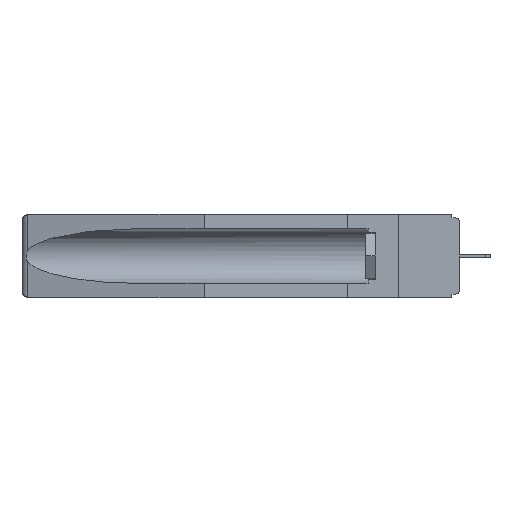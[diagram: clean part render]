
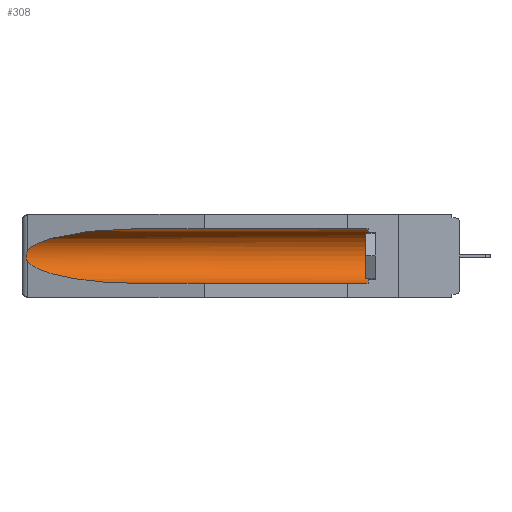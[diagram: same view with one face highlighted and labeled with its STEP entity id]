
A CAD part, left-side view. The second image highlights one B-rep face of the part: STEP entity #308.
In plain terms, the highlighted cylindrical face has radius 2.857 mm (diameter 5.715 mm), a partial arc.
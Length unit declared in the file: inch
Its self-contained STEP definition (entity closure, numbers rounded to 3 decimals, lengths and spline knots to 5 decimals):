
#35 = B_SPLINE_CURVE_WITH_KNOTS ( 'NONE', 3,
 ( #10363, #8998, #11764, #3675, #13115, #5022, #14441, #6374, #15782, #7714 ),
 .UNSPECIFIED., .F., .F.,
 ( 4, 2, 2, 2, 4 ),
 ( 0., 0.00029, 0.00058, 0.00087, 0.00117 ),
 .UNSPECIFIED. ) ;
#308 = ADVANCED_FACE ( 'NONE', ( #6206 ), #5786, .F. ) ;
#418 = ORIENTED_EDGE ( 'NONE', *, *, #5376, .T. ) ;
#482 = CARTESIAN_POINT ( 'NONE',  ( 0.155, 0.126, -0.284 ) ) ;
#918 = EDGE_CURVE ( 'NONE', #16884, #5468, #8248, .T. ) ;
#1491 = AXIS2_PLACEMENT_3D ( 'NONE', #14550, #6474, #15887 ) ;
#1547 = AXIS2_PLACEMENT_3D ( 'NONE', #2566, #2277, #8365 ) ;
#2277 = DIRECTION ( 'NONE',  ( 0., 1., 0. ) ) ;
#2528 =( BOUNDED_CURVE ( )  B_SPLINE_CURVE ( 3, ( #3553, #7594, #13040, #4959 ),
 .UNSPECIFIED., .F., .F. ) 
 B_SPLINE_CURVE_WITH_KNOTS ( ( 4, 4 ),
 ( 4.71239, 6.08839 ),
 .UNSPECIFIED. ) 
 CURVE ( )  GEOMETRIC_REPRESENTATION_ITEM ( )  RATIONAL_B_SPLINE_CURVE ( ( 1., 0.848, 0.848, 1. ) ) 
 REPRESENTATION_ITEM ( '' )  );
#2566 = CARTESIAN_POINT ( 'NONE',  ( 0.155, -0.30754, -0.1715 ) ) ;
#2602 = VERTEX_POINT ( 'NONE', #11420 ) ;
#3192 = CARTESIAN_POINT ( 'NONE',  ( 0.21114, 1.30732, -0.284 ) ) ;
#3553 = CARTESIAN_POINT ( 'NONE',  ( 0.155, 1.07973, -0.059 ) ) ;
#3661 = CARTESIAN_POINT ( 'NONE',  ( 0.155, 1.07973, -0.059 ) ) ;
#3675 = CARTESIAN_POINT ( 'NONE',  ( 0.2673, 1.5327, -0.16383 ) ) ;
#3689 = ORIENTED_EDGE ( 'NONE', *, *, #15114, .T. ) ;
#3740 = ORIENTED_EDGE ( 'NONE', *, *, #10896, .F. ) ;
#4436 = EDGE_CURVE ( 'NONE', #2602, #9497, #15044, .T. ) ;
#4898 = CARTESIAN_POINT ( 'NONE',  ( 0.25451, 1.48313, -0.24835 ) ) ;
#4959 = CARTESIAN_POINT ( 'NONE',  ( 0.26537, 1.52718, -0.14972 ) ) ;
#5022 = CARTESIAN_POINT ( 'NONE',  ( 0.2675, 1.53308, -0.17534 ) ) ;
#5091 = ORIENTED_EDGE ( 'NONE', *, *, #15191, .T. ) ;
#5251 = VERTEX_POINT ( 'NONE', #16597 ) ;
#5376 = EDGE_CURVE ( 'NONE', #5251, #16884, #35, .T. ) ;
#5468 = VERTEX_POINT ( 'NONE', #15959 ) ;
#5786 = CYLINDRICAL_SURFACE ( 'NONE', #1547, 0.1125 ) ;
#6206 = FACE_OUTER_BOUND ( 'NONE', #17355, .T. ) ;
#6374 = CARTESIAN_POINT ( 'NONE',  ( 0.26655, 1.53094, -0.18657 ) ) ;
#6474 = DIRECTION ( 'NONE',  ( 0., -1., 0. ) ) ;
#6485 = LINE ( 'NONE', #14271, #13250 ) ;
#7594 = CARTESIAN_POINT ( 'NONE',  ( 0.21114, 1.30732, -0.059 ) ) ;
#7714 = CARTESIAN_POINT ( 'NONE',  ( 0.26537, 1.52718, -0.19328 ) ) ;
#8248 =( BOUNDED_CURVE ( )  B_SPLINE_CURVE ( 3, ( #9800, #4898, #3192, #9164 ),
 .UNSPECIFIED., .F., .F. ) 
 B_SPLINE_CURVE_WITH_KNOTS ( ( 4, 4 ),
 ( 0.1948, 1.5708 ),
 .UNSPECIFIED. ) 
 CURVE ( )  GEOMETRIC_REPRESENTATION_ITEM ( )  RATIONAL_B_SPLINE_CURVE ( ( 1., 0.848, 0.848, 1. ) ) 
 REPRESENTATION_ITEM ( '' )  );
#8365 = DIRECTION ( 'NONE',  ( 0., 0., 1. ) ) ;
#8998 = CARTESIAN_POINT ( 'NONE',  ( 0.26597, 1.52961, -0.15275 ) ) ;
#9164 = CARTESIAN_POINT ( 'NONE',  ( 0.155, 1.07973, -0.284 ) ) ;
#9497 = VERTEX_POINT ( 'NONE', #3661 ) ;
#9800 = CARTESIAN_POINT ( 'NONE',  ( 0.26537, 1.52718, -0.19328 ) ) ;
#10363 = CARTESIAN_POINT ( 'NONE',  ( 0.26537, 1.52718, -0.14972 ) ) ;
#10792 = VERTEX_POINT ( 'NONE', #482 ) ;
#10896 = EDGE_CURVE ( 'NONE', #10792, #5468, #6485, .T. ) ;
#11054 = VECTOR ( 'NONE', #14106, 39.37008 ) ;
#11420 = CARTESIAN_POINT ( 'NONE',  ( 0.155, 0.126, -0.059 ) ) ;
#11439 = CIRCLE ( 'NONE', #1491, 0.1125 ) ;
#11764 = CARTESIAN_POINT ( 'NONE',  ( 0.26654, 1.53092, -0.15636 ) ) ;
#12186 = ORIENTED_EDGE ( 'NONE', *, *, #918, .T. ) ;
#13040 = CARTESIAN_POINT ( 'NONE',  ( 0.25451, 1.48313, -0.09465 ) ) ;
#13115 = CARTESIAN_POINT ( 'NONE',  ( 0.2675, 1.53308, -0.16763 ) ) ;
#13250 = VECTOR ( 'NONE', #15606, 39.37008 ) ;
#14063 = CARTESIAN_POINT ( 'NONE',  ( 0.155, -0.30754, -0.059 ) ) ;
#14106 = DIRECTION ( 'NONE',  ( 0., 1., 0. ) ) ;
#14271 = CARTESIAN_POINT ( 'NONE',  ( 0.155, -0.30754, -0.284 ) ) ;
#14441 = CARTESIAN_POINT ( 'NONE',  ( 0.2673, 1.53269, -0.17917 ) ) ;
#14550 = CARTESIAN_POINT ( 'NONE',  ( 0.155, 0.126, -0.1715 ) ) ;
#14930 = CARTESIAN_POINT ( 'NONE',  ( 0.26537, 1.52718, -0.19328 ) ) ;
#15044 = LINE ( 'NONE', #14063, #11054 ) ;
#15114 = EDGE_CURVE ( 'NONE', #9497, #5251, #2528, .T. ) ;
#15191 = EDGE_CURVE ( 'NONE', #10792, #2602, #11439, .T. ) ;
#15606 = DIRECTION ( 'NONE',  ( 0., 1., 0. ) ) ;
#15782 = CARTESIAN_POINT ( 'NONE',  ( 0.26597, 1.5296, -0.19026 ) ) ;
#15887 = DIRECTION ( 'NONE',  ( 0., 0., 1. ) ) ;
#15959 = CARTESIAN_POINT ( 'NONE',  ( 0.155, 1.07973, -0.284 ) ) ;
#16597 = CARTESIAN_POINT ( 'NONE',  ( 0.26537, 1.52718, -0.14972 ) ) ;
#16884 = VERTEX_POINT ( 'NONE', #14930 ) ;
#16912 = ORIENTED_EDGE ( 'NONE', *, *, #4436, .T. ) ;
#17355 = EDGE_LOOP ( 'NONE', ( #3689, #418, #12186, #3740, #5091, #16912 ) ) ;
